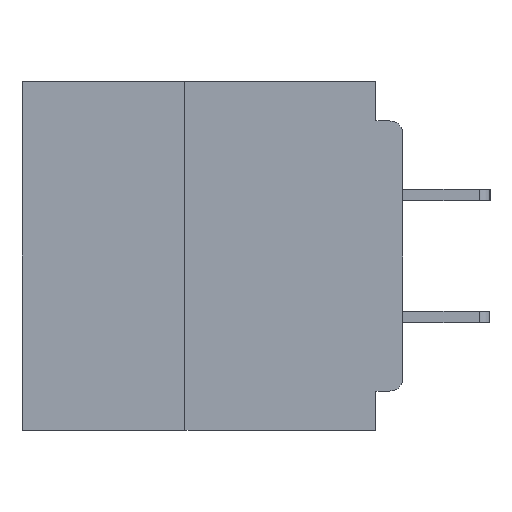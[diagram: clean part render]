
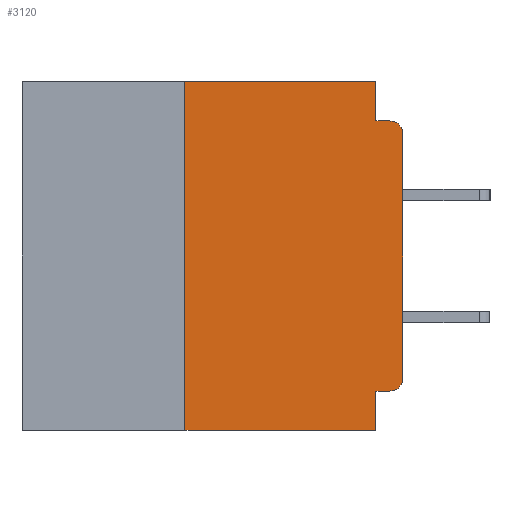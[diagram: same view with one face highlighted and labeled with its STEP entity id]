
A CAD part, left-side view. The second image highlights one B-rep face of the part: STEP entity #3120.
In plain terms, the highlighted planar face has unit normal (-1, 0, 0).
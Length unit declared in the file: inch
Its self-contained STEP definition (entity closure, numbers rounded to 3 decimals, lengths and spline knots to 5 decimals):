
#117 = VERTEX_POINT ( 'NONE', #27344 ) ;
#612 = VECTOR ( 'NONE', #3813, 39.37008 ) ;
#655 = EDGE_CURVE ( 'NONE', #28406, #55568, #14117, .T. ) ;
#1204 = AXIS2_PLACEMENT_3D ( 'NONE', #33496, #5424, #38202 ) ;
#2081 = VECTOR ( 'NONE', #27808, 39.37008 ) ;
#2172 = ORIENTED_EDGE ( 'NONE', *, *, #41721, .T. ) ;
#2540 = DIRECTION ( 'NONE',  ( 0., 1., 0. ) ) ;
#2792 = CARTESIAN_POINT ( 'NONE',  ( 0., 0.25, -0.4 ) ) ;
#3120 = ADVANCED_FACE ( 'NONE', ( #32943 ), #24784, .F. ) ;
#3189 = ORIENTED_EDGE ( 'NONE', *, *, #52751, .F. ) ;
#3633 = LINE ( 'NONE', #45750, #52032 ) ;
#3813 = DIRECTION ( 'NONE',  ( 0., 0., -1. ) ) ;
#3942 = VERTEX_POINT ( 'NONE', #49787 ) ;
#4639 = ORIENTED_EDGE ( 'NONE', *, *, #47556, .F. ) ;
#5424 = DIRECTION ( 'NONE',  ( -1., 0., 0. ) ) ;
#5683 = CARTESIAN_POINT ( 'NONE',  ( 0., 0.015, -0.06 ) ) ;
#8523 = CIRCLE ( 'NONE', #1204, 0.015 ) ;
#10400 = DIRECTION ( 'NONE',  ( 0., 0., -1. ) ) ;
#10494 = CARTESIAN_POINT ( 'NONE',  ( 0., 0.25, 0. ) ) ;
#11775 = VERTEX_POINT ( 'NONE', #54522 ) ;
#12465 = EDGE_LOOP ( 'NONE', ( #41639, #22446, #25438, #3189, #55386, #53784, #16773, #4639, #32633, #2172 ) ) ;
#12741 = EDGE_CURVE ( 'NONE', #11775, #3942, #55816, .T. ) ;
#14027 = AXIS2_PLACEMENT_3D ( 'NONE', #15384, #15598, #48356 ) ;
#14117 = LINE ( 'NONE', #16915, #39020 ) ;
#15285 = VERTEX_POINT ( 'NONE', #52423 ) ;
#15384 = CARTESIAN_POINT ( 'NONE',  ( 0., 0.437, 0. ) ) ;
#15598 = DIRECTION ( 'NONE',  ( 1., 0., 0. ) ) ;
#16165 = DIRECTION ( 'NONE',  ( 0., -1., 0. ) ) ;
#16773 = ORIENTED_EDGE ( 'NONE', *, *, #25345, .T. ) ;
#16915 = CARTESIAN_POINT ( 'NONE',  ( 0., 0., -0.045 ) ) ;
#19044 = VECTOR ( 'NONE', #35596, 39.37008 ) ;
#19718 = EDGE_CURVE ( 'NONE', #26458, #33569, #54923, .T. ) ;
#21381 = CARTESIAN_POINT ( 'NONE',  ( 0., 0., -0.355 ) ) ;
#22446 = ORIENTED_EDGE ( 'NONE', *, *, #40280, .T. ) ;
#22823 = DIRECTION ( 'NONE',  ( 0., 0., 1. ) ) ;
#23291 = CARTESIAN_POINT ( 'NONE',  ( 0., 0.015, -0.355 ) ) ;
#24784 = PLANE ( 'NONE',  #14027 ) ;
#25345 = EDGE_CURVE ( 'NONE', #26458, #43521, #3633, .T. ) ;
#25438 = ORIENTED_EDGE ( 'NONE', *, *, #655, .F. ) ;
#25550 = LINE ( 'NONE', #55802, #2081 ) ;
#26458 = VERTEX_POINT ( 'NONE', #40065 ) ;
#27007 = LINE ( 'NONE', #27406, #612 ) ;
#27344 = CARTESIAN_POINT ( 'NONE',  ( 0., 0.031, 0. ) ) ;
#27406 = CARTESIAN_POINT ( 'NONE',  ( 0., 0.031, 0. ) ) ;
#27808 = DIRECTION ( 'NONE',  ( 0., -1., 0. ) ) ;
#27886 = CARTESIAN_POINT ( 'NONE',  ( 0., 0.031, -0.4 ) ) ;
#28406 = VERTEX_POINT ( 'NONE', #50688 ) ;
#29484 = CARTESIAN_POINT ( 'NONE',  ( 0., 0.015, -0.045 ) ) ;
#30409 = VERTEX_POINT ( 'NONE', #23291 ) ;
#30953 = VECTOR ( 'NONE', #22823, 39.37008 ) ;
#32507 = LINE ( 'NONE', #21381, #54467 ) ;
#32633 = ORIENTED_EDGE ( 'NONE', *, *, #39278, .F. ) ;
#32943 = FACE_OUTER_BOUND ( 'NONE', #12465, .T. ) ;
#33496 = CARTESIAN_POINT ( 'NONE',  ( 0., 0.015, -0.34 ) ) ;
#33569 = VERTEX_POINT ( 'NONE', #10494 ) ;
#35596 = DIRECTION ( 'NONE',  ( 0., 0., 1. ) ) ;
#36317 = EDGE_CURVE ( 'NONE', #33569, #117, #25550, .T. ) ;
#37233 = VECTOR ( 'NONE', #55894, 39.37008 ) ;
#38202 = DIRECTION ( 'NONE',  ( 0., 0., -1. ) ) ;
#38482 = DIRECTION ( 'NONE',  ( -1., 0., 0. ) ) ;
#38697 = LINE ( 'NONE', #27886, #37233 ) ;
#39020 = VECTOR ( 'NONE', #16165, 39.37008 ) ;
#39278 = EDGE_CURVE ( 'NONE', #30409, #15285, #32507, .T. ) ;
#40065 = CARTESIAN_POINT ( 'NONE',  ( 0., 0.25, -0.4 ) ) ;
#40280 = EDGE_CURVE ( 'NONE', #3942, #55568, #57955, .T. ) ;
#41639 = ORIENTED_EDGE ( 'NONE', *, *, #12741, .T. ) ;
#41721 = EDGE_CURVE ( 'NONE', #30409, #11775, #8523, .T. ) ;
#43521 = VERTEX_POINT ( 'NONE', #46210 ) ;
#44730 = AXIS2_PLACEMENT_3D ( 'NONE', #5683, #38482, #10400 ) ;
#45750 = CARTESIAN_POINT ( 'NONE',  ( 0., 0.437, -0.4 ) ) ;
#46210 = CARTESIAN_POINT ( 'NONE',  ( 0., 0.031, -0.4 ) ) ;
#47556 = EDGE_CURVE ( 'NONE', #15285, #43521, #38697, .T. ) ;
#48356 = DIRECTION ( 'NONE',  ( 0., 0., -1. ) ) ;
#49787 = CARTESIAN_POINT ( 'NONE',  ( 0., 0., -0.06 ) ) ;
#50688 = CARTESIAN_POINT ( 'NONE',  ( 0., 0.031, -0.045 ) ) ;
#52032 = VECTOR ( 'NONE', #55146, 39.37008 ) ;
#52423 = CARTESIAN_POINT ( 'NONE',  ( 0., 0.031, -0.355 ) ) ;
#52751 = EDGE_CURVE ( 'NONE', #117, #28406, #27007, .T. ) ;
#53784 = ORIENTED_EDGE ( 'NONE', *, *, #19718, .F. ) ;
#54467 = VECTOR ( 'NONE', #2540, 39.37008 ) ;
#54522 = CARTESIAN_POINT ( 'NONE',  ( 0., 0., -0.34 ) ) ;
#54923 = LINE ( 'NONE', #2792, #19044 ) ;
#55146 = DIRECTION ( 'NONE',  ( 0., -1., 0. ) ) ;
#55386 = ORIENTED_EDGE ( 'NONE', *, *, #36317, .F. ) ;
#55568 = VERTEX_POINT ( 'NONE', #29484 ) ;
#55802 = CARTESIAN_POINT ( 'NONE',  ( 0., 0.437, 0. ) ) ;
#55816 = LINE ( 'NONE', #60223, #30953 ) ;
#55894 = DIRECTION ( 'NONE',  ( 0., 0., -1. ) ) ;
#57955 = CIRCLE ( 'NONE', #44730, 0.015 ) ;
#60223 = CARTESIAN_POINT ( 'NONE',  ( 0., 0., 0. ) ) ;
